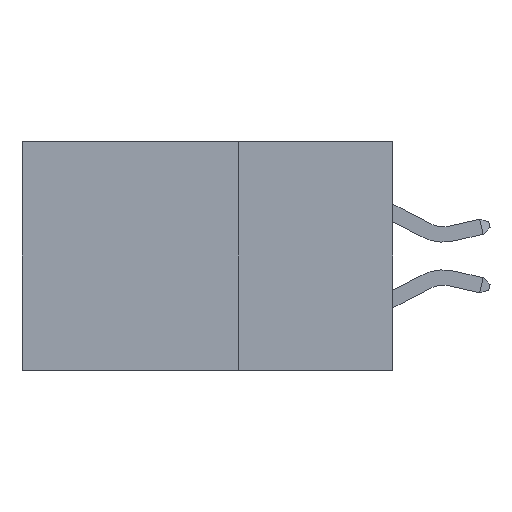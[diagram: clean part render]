
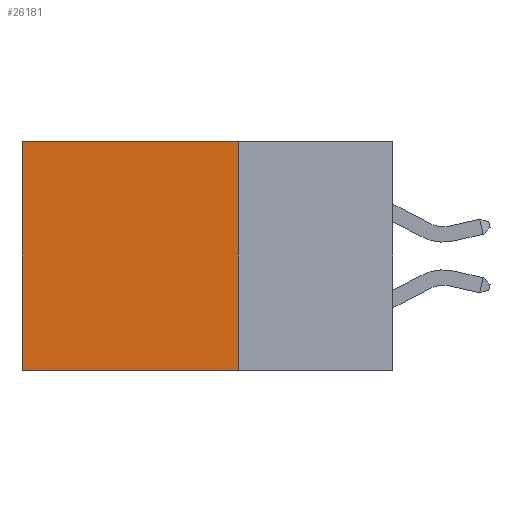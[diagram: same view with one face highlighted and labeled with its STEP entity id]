
A CAD part, left-side view. The second image highlights one B-rep face of the part: STEP entity #26181.
In plain terms, the highlighted planar face has unit normal (-1, 0, 0).
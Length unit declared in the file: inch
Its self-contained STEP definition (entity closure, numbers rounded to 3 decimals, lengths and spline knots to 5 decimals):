
#263 = EDGE_CURVE ( 'NONE', #6510, #11212, #28165, .T. ) ;
#1109 = AXIS2_PLACEMENT_3D ( 'NONE', #11275, #15767, #2443 ) ;
#1182 = LINE ( 'NONE', #27757, #24646 ) ;
#1720 = LINE ( 'NONE', #17135, #12871 ) ;
#2034 = EDGE_LOOP ( 'NONE', ( #16573, #21306, #24001, #19119 ) ) ;
#2145 = VECTOR ( 'NONE', #4765, 39.37008 ) ;
#2177 = CARTESIAN_POINT ( 'NONE',  ( 0.2875, 0.25, 0. ) ) ;
#2443 = DIRECTION ( 'NONE',  ( 0., 0., -1. ) ) ;
#4765 = DIRECTION ( 'NONE',  ( 0., 1., 0. ) ) ;
#4853 = CARTESIAN_POINT ( 'NONE',  ( 0.2875, 0.25, 0. ) ) ;
#5714 = CARTESIAN_POINT ( 'NONE',  ( 0.2875, 0.25, -0.37 ) ) ;
#6016 = DIRECTION ( 'NONE',  ( 0., 1., 0. ) ) ;
#6510 = VERTEX_POINT ( 'NONE', #2177 ) ;
#7029 = FACE_OUTER_BOUND ( 'NONE', #2034, .T. ) ;
#8034 = LINE ( 'NONE', #20289, #2145 ) ;
#9288 = EDGE_CURVE ( 'NONE', #6510, #18020, #8034, .T. ) ;
#10643 = VECTOR ( 'NONE', #22947, 39.37008 ) ;
#10816 = CARTESIAN_POINT ( 'NONE',  ( 0.2875, 0.6, -0.37 ) ) ;
#11212 = VERTEX_POINT ( 'NONE', #5714 ) ;
#11275 = CARTESIAN_POINT ( 'NONE',  ( 0.2875, 0.25, 0. ) ) ;
#12871 = VECTOR ( 'NONE', #6016, 39.37008 ) ;
#13548 = PLANE ( 'NONE',  #1109 ) ;
#15767 = DIRECTION ( 'NONE',  ( 1., 0., 0. ) ) ;
#16573 = ORIENTED_EDGE ( 'NONE', *, *, #26162, .T. ) ;
#17135 = CARTESIAN_POINT ( 'NONE',  ( 0.2875, 0.25, -0.37 ) ) ;
#18020 = VERTEX_POINT ( 'NONE', #22657 ) ;
#19119 = ORIENTED_EDGE ( 'NONE', *, *, #9288, .T. ) ;
#20289 = CARTESIAN_POINT ( 'NONE',  ( 0.2875, 0.25, 0. ) ) ;
#21306 = ORIENTED_EDGE ( 'NONE', *, *, #23692, .F. ) ;
#22160 = DIRECTION ( 'NONE',  ( 0., 0., -1. ) ) ;
#22657 = CARTESIAN_POINT ( 'NONE',  ( 0.2875, 0.6, 0. ) ) ;
#22947 = DIRECTION ( 'NONE',  ( 0., 0., -1. ) ) ;
#23692 = EDGE_CURVE ( 'NONE', #11212, #24984, #1720, .T. ) ;
#24001 = ORIENTED_EDGE ( 'NONE', *, *, #263, .F. ) ;
#24646 = VECTOR ( 'NONE', #22160, 39.37008 ) ;
#24984 = VERTEX_POINT ( 'NONE', #10816 ) ;
#26162 = EDGE_CURVE ( 'NONE', #18020, #24984, #1182, .T. ) ;
#26181 = ADVANCED_FACE ( 'NONE', ( #7029 ), #13548, .F. ) ;
#27757 = CARTESIAN_POINT ( 'NONE',  ( 0.2875, 0.6, 0. ) ) ;
#28165 = LINE ( 'NONE', #4853, #10643 ) ;
